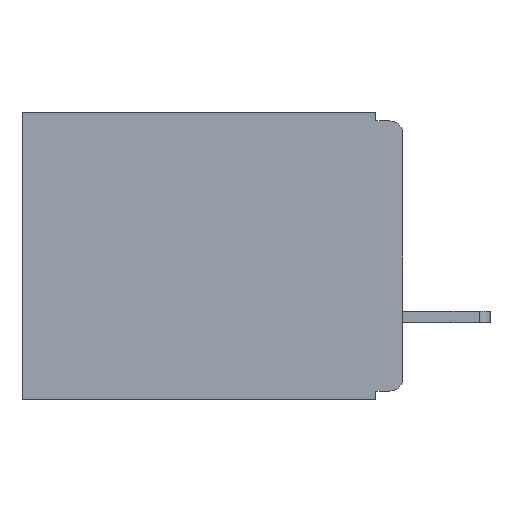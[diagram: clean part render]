
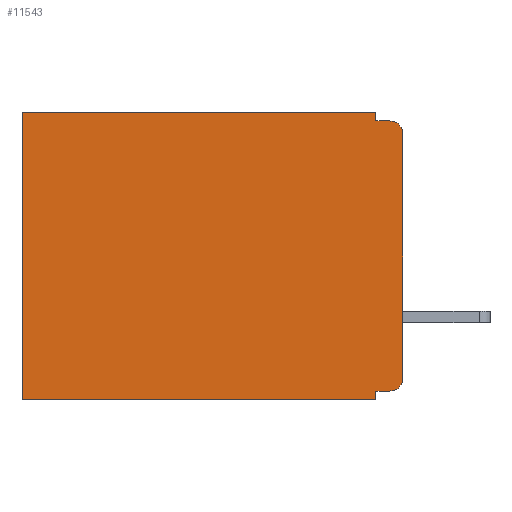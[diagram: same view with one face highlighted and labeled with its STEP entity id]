
A CAD part, left-side view. The second image highlights one B-rep face of the part: STEP entity #11543.
In plain terms, the highlighted planar face has unit normal (-1, 0, 0).
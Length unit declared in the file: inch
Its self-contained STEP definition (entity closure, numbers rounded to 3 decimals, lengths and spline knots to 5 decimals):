
#90 = VECTOR ( 'NONE', #2259, 39.37008 ) ;
#140 = CARTESIAN_POINT ( 'NONE',  ( 0.3, 0.015, -0.01 ) ) ;
#325 = CARTESIAN_POINT ( 'NONE',  ( 0.3, 0.015, -0.305 ) ) ;
#364 = CARTESIAN_POINT ( 'NONE',  ( 0.3, 0., -0.305 ) ) ;
#1587 = EDGE_LOOP ( 'NONE', ( #26938, #10332, #9077, #14359, #3149, #12127, #17419, #26329, #18092, #20501 ) ) ;
#1739 = VECTOR ( 'NONE', #18667, 39.37008 ) ;
#2222 = EDGE_CURVE ( 'NONE', #26111, #13914, #14957, .T. ) ;
#2259 = DIRECTION ( 'NONE',  ( 0., 0., -1. ) ) ;
#2402 = CARTESIAN_POINT ( 'NONE',  ( 0.3, 0.015, -0.32 ) ) ;
#3011 = DIRECTION ( 'NONE',  ( 0., 0., -1. ) ) ;
#3139 = AXIS2_PLACEMENT_3D ( 'NONE', #24243, #26802, #11239 ) ;
#3149 = ORIENTED_EDGE ( 'NONE', *, *, #28745, .T. ) ;
#3597 = VECTOR ( 'NONE', #30649, 39.37008 ) ;
#3647 = VECTOR ( 'NONE', #26700, 39.37008 ) ;
#4124 = CIRCLE ( 'NONE', #16846, 0.015 ) ;
#4217 = VECTOR ( 'NONE', #14847, 39.37008 ) ;
#4218 = FACE_OUTER_BOUND ( 'NONE', #1587, .T. ) ;
#6029 = PLANE ( 'NONE',  #3139 ) ;
#6267 = DIRECTION ( 'NONE',  ( -1., 0., 0. ) ) ;
#7453 = LINE ( 'NONE', #13282, #12709 ) ;
#7743 = CIRCLE ( 'NONE', #25442, 0.015 ) ;
#8085 = VECTOR ( 'NONE', #15337, 39.37008 ) ;
#8731 = LINE ( 'NONE', #31393, #1739 ) ;
#9077 = ORIENTED_EDGE ( 'NONE', *, *, #17813, .F. ) ;
#9354 = VERTEX_POINT ( 'NONE', #27498 ) ;
#9624 = VERTEX_POINT ( 'NONE', #364 ) ;
#9643 = EDGE_CURVE ( 'NONE', #26724, #27483, #24424, .T. ) ;
#10332 = ORIENTED_EDGE ( 'NONE', *, *, #13396, .T. ) ;
#10918 = CARTESIAN_POINT ( 'NONE',  ( 0.3, 0.031, -0.32 ) ) ;
#10980 = CARTESIAN_POINT ( 'NONE',  ( 0.3, 0.437, -0.33 ) ) ;
#11239 = DIRECTION ( 'NONE',  ( 0., 0., -1. ) ) ;
#11543 = ADVANCED_FACE ( 'NONE', ( #4218 ), #6029, .F. ) ;
#12127 = ORIENTED_EDGE ( 'NONE', *, *, #32482, .T. ) ;
#12709 = VECTOR ( 'NONE', #15877, 39.37008 ) ;
#12776 = EDGE_CURVE ( 'NONE', #15268, #9624, #26480, .T. ) ;
#13282 = CARTESIAN_POINT ( 'NONE',  ( 0.3, 0., 0. ) ) ;
#13396 = EDGE_CURVE ( 'NONE', #15268, #21562, #7743, .T. ) ;
#13555 = CARTESIAN_POINT ( 'NONE',  ( 0.3, 0., -0.33 ) ) ;
#13638 = CARTESIAN_POINT ( 'NONE',  ( 0.3, 0., -0.32 ) ) ;
#13860 = VERTEX_POINT ( 'NONE', #23870 ) ;
#13914 = VERTEX_POINT ( 'NONE', #10980 ) ;
#14359 = ORIENTED_EDGE ( 'NONE', *, *, #21422, .F. ) ;
#14587 = CARTESIAN_POINT ( 'NONE',  ( 0.3, 0., -0.33 ) ) ;
#14847 = DIRECTION ( 'NONE',  ( 0., -1., 0. ) ) ;
#14957 = LINE ( 'NONE', #14587, #8085 ) ;
#15105 = CARTESIAN_POINT ( 'NONE',  ( 0.3, 0.031, -0.01 ) ) ;
#15268 = VERTEX_POINT ( 'NONE', #16935 ) ;
#15337 = DIRECTION ( 'NONE',  ( 0., 1., 0. ) ) ;
#15877 = DIRECTION ( 'NONE',  ( 0., 1., 0. ) ) ;
#16154 = DIRECTION ( 'NONE',  ( 0., 0., -1. ) ) ;
#16846 = AXIS2_PLACEMENT_3D ( 'NONE', #325, #18634, #3011 ) ;
#16935 = CARTESIAN_POINT ( 'NONE',  ( 0.3, 0., -0.025 ) ) ;
#17226 = VERTEX_POINT ( 'NONE', #15105 ) ;
#17419 = ORIENTED_EDGE ( 'NONE', *, *, #2222, .F. ) ;
#17431 = LINE ( 'NONE', #25622, #3597 ) ;
#17463 = EDGE_CURVE ( 'NONE', #27483, #26111, #8731, .T. ) ;
#17714 = CARTESIAN_POINT ( 'NONE',  ( 0.3, 0.031, -0.33 ) ) ;
#17813 = EDGE_CURVE ( 'NONE', #17226, #21562, #32416, .T. ) ;
#18092 = ORIENTED_EDGE ( 'NONE', *, *, #9643, .F. ) ;
#18634 = DIRECTION ( 'NONE',  ( -1., 0., 0. ) ) ;
#18667 = DIRECTION ( 'NONE',  ( 0., 0., -1. ) ) ;
#18779 = VECTOR ( 'NONE', #16154, 39.37008 ) ;
#19887 = EDGE_CURVE ( 'NONE', #26724, #9624, #4124, .T. ) ;
#20135 = CARTESIAN_POINT ( 'NONE',  ( 0.3, 0., -0.01 ) ) ;
#20501 = ORIENTED_EDGE ( 'NONE', *, *, #19887, .T. ) ;
#21422 = EDGE_CURVE ( 'NONE', #13860, #17226, #17431, .T. ) ;
#21562 = VERTEX_POINT ( 'NONE', #140 ) ;
#21853 = CARTESIAN_POINT ( 'NONE',  ( 0.3, 0.015, -0.025 ) ) ;
#23870 = CARTESIAN_POINT ( 'NONE',  ( 0.3, 0.031, 0. ) ) ;
#24243 = CARTESIAN_POINT ( 'NONE',  ( 0.3, 0., -0.33 ) ) ;
#24424 = LINE ( 'NONE', #13638, #3647 ) ;
#24463 = DIRECTION ( 'NONE',  ( 0., 0., -1. ) ) ;
#25442 = AXIS2_PLACEMENT_3D ( 'NONE', #21853, #6267, #24463 ) ;
#25622 = CARTESIAN_POINT ( 'NONE',  ( 0.3, 0.031, 0. ) ) ;
#25634 = CARTESIAN_POINT ( 'NONE',  ( 0.3, 0.437, -0.33 ) ) ;
#26111 = VERTEX_POINT ( 'NONE', #17714 ) ;
#26329 = ORIENTED_EDGE ( 'NONE', *, *, #17463, .F. ) ;
#26480 = LINE ( 'NONE', #13555, #18779 ) ;
#26700 = DIRECTION ( 'NONE',  ( 0., 1., 0. ) ) ;
#26724 = VERTEX_POINT ( 'NONE', #2402 ) ;
#26802 = DIRECTION ( 'NONE',  ( 1., 0., 0. ) ) ;
#26938 = ORIENTED_EDGE ( 'NONE', *, *, #12776, .F. ) ;
#27026 = LINE ( 'NONE', #25634, #90 ) ;
#27483 = VERTEX_POINT ( 'NONE', #10918 ) ;
#27498 = CARTESIAN_POINT ( 'NONE',  ( 0.3, 0.437, 0. ) ) ;
#28745 = EDGE_CURVE ( 'NONE', #13860, #9354, #7453, .T. ) ;
#30649 = DIRECTION ( 'NONE',  ( 0., 0., -1. ) ) ;
#31393 = CARTESIAN_POINT ( 'NONE',  ( 0.3, 0.031, -0.33 ) ) ;
#32416 = LINE ( 'NONE', #20135, #4217 ) ;
#32482 = EDGE_CURVE ( 'NONE', #9354, #13914, #27026, .T. ) ;
